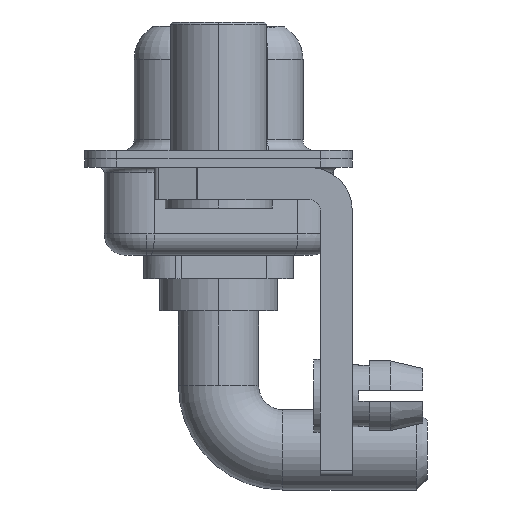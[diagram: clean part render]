
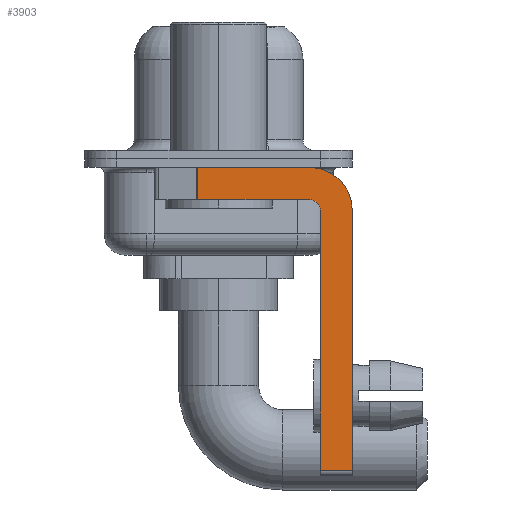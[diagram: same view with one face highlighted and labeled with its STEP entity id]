
A CAD part, left-side view. The second image highlights one B-rep face of the part: STEP entity #3903.
In plain terms, the highlighted planar face has unit normal (-1, 0, 0).
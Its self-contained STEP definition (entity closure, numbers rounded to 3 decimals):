
#59 = LINE ( 'NONE', #9715, #10523 ) ;
#97 = CARTESIAN_POINT ( 'NONE',  ( -2.9, -4.75, -2.4 ) ) ;
#108 = VERTEX_POINT ( 'NONE', #13866 ) ;
#419 = DIRECTION ( 'NONE',  ( 0., 0., 1. ) ) ;
#535 = VECTOR ( 'NONE', #5428, 1000. ) ;
#640 = EDGE_CURVE ( 'NONE', #7339, #108, #8877, .T. ) ;
#935 = ORIENTED_EDGE ( 'NONE', *, *, #3974, .T. ) ;
#1033 = VERTEX_POINT ( 'NONE', #15030 ) ;
#1045 = VECTOR ( 'NONE', #13828, 1000. ) ;
#1076 = ORIENTED_EDGE ( 'NONE', *, *, #13886, .F. ) ;
#1375 = PLANE ( 'NONE',  #7399 ) ;
#1424 = DIRECTION ( 'NONE',  ( 1., 0., 0. ) ) ;
#1591 = CARTESIAN_POINT ( 'NONE',  ( -2.9, -4.25, -2.4 ) ) ;
#1884 = EDGE_CURVE ( 'NONE', #14405, #12570, #13889, .T. ) ;
#2010 = AXIS2_PLACEMENT_3D ( 'NONE', #1591, #1424, #6345 ) ;
#2346 = DIRECTION ( 'NONE',  ( 0., 0., -1. ) ) ;
#2667 = DIRECTION ( 'NONE',  ( 0., 0., -1. ) ) ;
#2795 = EDGE_CURVE ( 'NONE', #1033, #108, #3553, .T. ) ;
#3038 = CARTESIAN_POINT ( 'NONE',  ( -2.9, 0.978, -0.4 ) ) ;
#3046 = EDGE_CURVE ( 'NONE', #9186, #11896, #4266, .T. ) ;
#3462 = DIRECTION ( 'NONE',  ( 0., 1., 0. ) ) ;
#3553 = LINE ( 'NONE', #13346, #12287 ) ;
#3903 = ADVANCED_FACE ( 'NONE', ( #5076 ), #1375, .F. ) ;
#3974 = EDGE_CURVE ( 'NONE', #9186, #13109, #4439, .T. ) ;
#4060 = DIRECTION ( 'NONE',  ( 0., 0., 1. ) ) ;
#4146 = CARTESIAN_POINT ( 'NONE',  ( -2.9, -4.25, -14.55 ) ) ;
#4266 = LINE ( 'NONE', #6914, #5915 ) ;
#4439 = LINE ( 'NONE', #7825, #1045 ) ;
#5076 = FACE_OUTER_BOUND ( 'NONE', #8054, .T. ) ;
#5270 = CARTESIAN_POINT ( 'NONE',  ( -2.9, -4.25, -1.9 ) ) ;
#5428 = DIRECTION ( 'NONE',  ( 0., -1., 0. ) ) ;
#5637 = DIRECTION ( 'NONE',  ( 0., -1., 0. ) ) ;
#5915 = VECTOR ( 'NONE', #5637, 1000. ) ;
#6345 = DIRECTION ( 'NONE',  ( 0., 0., -1. ) ) ;
#6382 = CARTESIAN_POINT ( 'NONE',  ( -2.9, 0.978, -1.9 ) ) ;
#6914 = CARTESIAN_POINT ( 'NONE',  ( -2.9, 3., -0.4 ) ) ;
#6989 = AXIS2_PLACEMENT_3D ( 'NONE', #9193, #12634, #4060 ) ;
#7339 = VERTEX_POINT ( 'NONE', #15272 ) ;
#7399 = AXIS2_PLACEMENT_3D ( 'NONE', #14877, #13668, #2667 ) ;
#7675 = LINE ( 'NONE', #14964, #8906 ) ;
#7700 = ORIENTED_EDGE ( 'NONE', *, *, #3046, .F. ) ;
#7798 = ORIENTED_EDGE ( 'NONE', *, *, #10351, .F. ) ;
#7825 = CARTESIAN_POINT ( 'NONE',  ( -2.9, 0.978, -1.9 ) ) ;
#8054 = EDGE_LOOP ( 'NONE', ( #7700, #935, #1076, #9191, #7798, #10876, #13627, #10172 ) ) ;
#8877 = LINE ( 'NONE', #4146, #535 ) ;
#8906 = VECTOR ( 'NONE', #419, 1000. ) ;
#9069 = EDGE_CURVE ( 'NONE', #11896, #1033, #13030, .T. ) ;
#9186 = VERTEX_POINT ( 'NONE', #3038 ) ;
#9191 = ORIENTED_EDGE ( 'NONE', *, *, #1884, .F. ) ;
#9193 = CARTESIAN_POINT ( 'NONE',  ( -2.9, -4.25, -2.4 ) ) ;
#9715 = CARTESIAN_POINT ( 'NONE',  ( -2.9, -4.25, -1.9 ) ) ;
#10172 = ORIENTED_EDGE ( 'NONE', *, *, #9069, .F. ) ;
#10351 = EDGE_CURVE ( 'NONE', #7339, #14405, #7675, .T. ) ;
#10382 = CARTESIAN_POINT ( 'NONE',  ( -2.9, -4.25, -0.4 ) ) ;
#10523 = VECTOR ( 'NONE', #3462, 1000. ) ;
#10876 = ORIENTED_EDGE ( 'NONE', *, *, #640, .T. ) ;
#11896 = VERTEX_POINT ( 'NONE', #10382 ) ;
#12287 = VECTOR ( 'NONE', #2346, 1000. ) ;
#12570 = VERTEX_POINT ( 'NONE', #5270 ) ;
#12634 = DIRECTION ( 'NONE',  ( -1., 0., 0. ) ) ;
#13030 = CIRCLE ( 'NONE', #2010, 2. ) ;
#13109 = VERTEX_POINT ( 'NONE', #6382 ) ;
#13346 = CARTESIAN_POINT ( 'NONE',  ( -2.9, -6.25, -2.4 ) ) ;
#13627 = ORIENTED_EDGE ( 'NONE', *, *, #2795, .F. ) ;
#13668 = DIRECTION ( 'NONE',  ( 1., 0., 0. ) ) ;
#13828 = DIRECTION ( 'NONE',  ( 0., 0., -1. ) ) ;
#13866 = CARTESIAN_POINT ( 'NONE',  ( -2.9, -6.25, -14.55 ) ) ;
#13886 = EDGE_CURVE ( 'NONE', #12570, #13109, #59, .T. ) ;
#13889 = CIRCLE ( 'NONE', #6989, 0.5 ) ;
#14405 = VERTEX_POINT ( 'NONE', #97 ) ;
#14877 = CARTESIAN_POINT ( 'NONE',  ( -2.9, -4.25, -2.4 ) ) ;
#14964 = CARTESIAN_POINT ( 'NONE',  ( -2.9, -4.75, -14.8 ) ) ;
#15030 = CARTESIAN_POINT ( 'NONE',  ( -2.9, -6.25, -2.4 ) ) ;
#15272 = CARTESIAN_POINT ( 'NONE',  ( -2.9, -4.75, -14.55 ) ) ;
